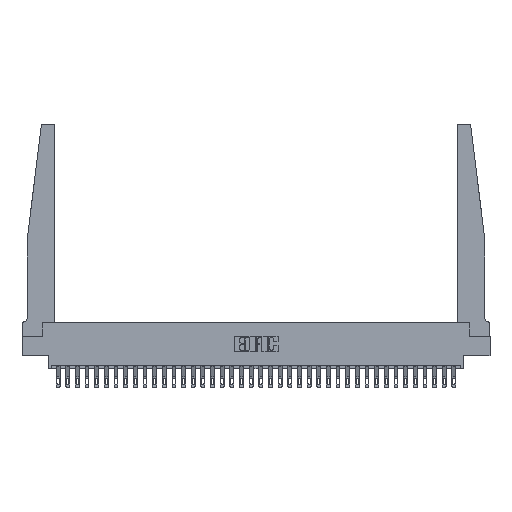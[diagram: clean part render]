
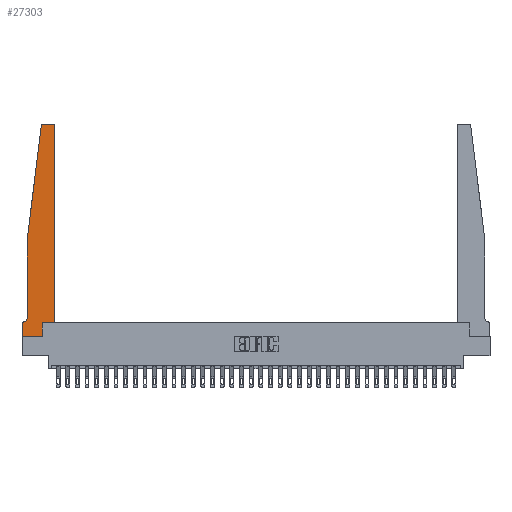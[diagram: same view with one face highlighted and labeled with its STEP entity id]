
A CAD part, top view. The second image highlights one B-rep face of the part: STEP entity #27303.
In plain terms, the highlighted planar face has unit normal (0, 0, 1).
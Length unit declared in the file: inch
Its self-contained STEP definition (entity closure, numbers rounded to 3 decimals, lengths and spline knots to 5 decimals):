
#251 = DIRECTION ( 'NONE',  ( -1., 0., 0. ) ) ;
#443 = ORIENTED_EDGE ( 'NONE', *, *, #30483, .T. ) ;
#712 = VECTOR ( 'NONE', #25133, 39.37008 ) ;
#1292 = ORIENTED_EDGE ( 'NONE', *, *, #17902, .T. ) ;
#2018 = CARTESIAN_POINT ( 'NONE',  ( 0.27653, 2.72, 0.37 ) ) ;
#2339 = DIRECTION ( 'NONE',  ( 0., 0., 1. ) ) ;
#2345 = LINE ( 'NONE', #12556, #712 ) ;
#2623 = LINE ( 'NONE', #23044, #21802 ) ;
#2804 = CARTESIAN_POINT ( 'NONE',  ( 0.27653, 2.75, 0.37 ) ) ;
#2879 = EDGE_CURVE ( 'NONE', #19835, #14535, #21771, .T. ) ;
#3100 = EDGE_CURVE ( 'NONE', #9063, #32251, #10012, .T. ) ;
#3103 = VECTOR ( 'NONE', #7460, 39.37008 ) ;
#3118 = CARTESIAN_POINT ( 'NONE',  ( 0.425, 0.18, 0.37 ) ) ;
#3523 = VERTEX_POINT ( 'NONE', #20181 ) ;
#3571 = FACE_OUTER_BOUND ( 'NONE', #21471, .T. ) ;
#3615 = LINE ( 'NONE', #13838, #16624 ) ;
#3735 = VECTOR ( 'NONE', #15206, 39.37008 ) ;
#4100 = DIRECTION ( 'NONE',  ( 1., 0., 0. ) ) ;
#4195 = ORIENTED_EDGE ( 'NONE', *, *, #2879, .T. ) ;
#4734 = EDGE_CURVE ( 'NONE', #32251, #16975, #20348, .T. ) ;
#4829 = EDGE_CURVE ( 'NONE', #31759, #8636, #2623, .T. ) ;
#5048 = CARTESIAN_POINT ( 'NONE',  ( 0.24675, 2.72367, 0.37 ) ) ;
#5418 = ORIENTED_EDGE ( 'NONE', *, *, #32273, .T. ) ;
#5441 = ORIENTED_EDGE ( 'NONE', *, *, #25520, .T. ) ;
#6023 = CARTESIAN_POINT ( 'NONE',  ( 0.2605, 0., 0.37 ) ) ;
#6103 = CARTESIAN_POINT ( 'NONE',  ( 0., 0., 0.37 ) ) ;
#6247 = DIRECTION ( 'NONE',  ( 1., 0., 0. ) ) ;
#6386 = CIRCLE ( 'NONE', #14946, 0.05 ) ;
#7021 = ORIENTED_EDGE ( 'NONE', *, *, #22419, .T. ) ;
#7460 = DIRECTION ( 'NONE',  ( 0., -1., 0. ) ) ;
#8636 = VERTEX_POINT ( 'NONE', #30446 ) ;
#8639 = DIRECTION ( 'NONE',  ( 0., 1., 0. ) ) ;
#8649 = CIRCLE ( 'NONE', #16198, 0.03 ) ;
#8762 = CARTESIAN_POINT ( 'NONE',  ( 0., 0.1875, 0.37 ) ) ;
#9031 = VECTOR ( 'NONE', #4100, 39.37008 ) ;
#9063 = VERTEX_POINT ( 'NONE', #5048 ) ;
#9319 = DIRECTION ( 'NONE',  ( -1., 0., 0. ) ) ;
#9564 = EDGE_CURVE ( 'NONE', #14535, #9063, #8649, .T. ) ;
#10012 = LINE ( 'NONE', #30470, #3735 ) ;
#10128 = DIRECTION ( 'NONE',  ( 0., 0., -1. ) ) ;
#10721 = VERTEX_POINT ( 'NONE', #28038 ) ;
#10940 = CARTESIAN_POINT ( 'NONE',  ( 0.395, 2.72, 0.37 ) ) ;
#12046 = CARTESIAN_POINT ( 'NONE',  ( 0.25, 2.75, 0.37 ) ) ;
#12157 = CARTESIAN_POINT ( 'NONE',  ( 0.065, 0.1875, 0.37 ) ) ;
#12234 = DIRECTION ( 'NONE',  ( 1., 0., 0. ) ) ;
#12323 = CARTESIAN_POINT ( 'NONE',  ( 0., 0., 0.37 ) ) ;
#12491 = CARTESIAN_POINT ( 'NONE',  ( 0.015, 0.2375, 0.37 ) ) ;
#12556 = CARTESIAN_POINT ( 'NONE',  ( 0.425, 0.18, 0.37 ) ) ;
#12563 = CARTESIAN_POINT ( 'NONE',  ( 0.395, 2.75, 0.37 ) ) ;
#13838 = CARTESIAN_POINT ( 'NONE',  ( 0., 0., 0.37 ) ) ;
#13849 = ORIENTED_EDGE ( 'NONE', *, *, #4829, .T. ) ;
#14535 = VERTEX_POINT ( 'NONE', #2804 ) ;
#14572 = DIRECTION ( 'NONE',  ( -1., 0., 0. ) ) ;
#14625 = ORIENTED_EDGE ( 'NONE', *, *, #17538, .T. ) ;
#14946 = AXIS2_PLACEMENT_3D ( 'NONE', #12491, #10128, #251 ) ;
#15206 = DIRECTION ( 'NONE',  ( -0.122, -0.992, 0. ) ) ;
#15298 = DIRECTION ( 'NONE',  ( 0., 0., 1. ) ) ;
#15834 = LINE ( 'NONE', #3118, #21204 ) ;
#16198 = AXIS2_PLACEMENT_3D ( 'NONE', #2018, #2339, #12234 ) ;
#16624 = VECTOR ( 'NONE', #19010, 39.37008 ) ;
#16975 = VERTEX_POINT ( 'NONE', #20726 ) ;
#17502 = CIRCLE ( 'NONE', #26073, 0.03 ) ;
#17538 = EDGE_CURVE ( 'NONE', #28084, #3523, #15834, .T. ) ;
#17902 = EDGE_CURVE ( 'NONE', #3523, #19835, #17502, .T. ) ;
#18138 = DIRECTION ( 'NONE',  ( 1., 0., 0. ) ) ;
#18936 = VERTEX_POINT ( 'NONE', #12323 ) ;
#19010 = DIRECTION ( 'NONE',  ( 0., -1., 0. ) ) ;
#19142 = PLANE ( 'NONE',  #25193 ) ;
#19619 = VECTOR ( 'NONE', #14572, 39.37008 ) ;
#19635 = CARTESIAN_POINT ( 'NONE',  ( 0.015, 0.1875, 0.37 ) ) ;
#19835 = VERTEX_POINT ( 'NONE', #12563 ) ;
#20181 = CARTESIAN_POINT ( 'NONE',  ( 0.425, 2.72, 0.37 ) ) ;
#20348 = LINE ( 'NONE', #20517, #3103 ) ;
#20517 = CARTESIAN_POINT ( 'NONE',  ( 0.065, 1.25, 0.37 ) ) ;
#20726 = CARTESIAN_POINT ( 'NONE',  ( 0.065, 0.2375, 0.37 ) ) ;
#20914 = LINE ( 'NONE', #6103, #9031 ) ;
#21204 = VECTOR ( 'NONE', #23559, 39.37008 ) ;
#21471 = EDGE_LOOP ( 'NONE', ( #4195, #22852, #27718, #32979, #5441, #5418, #24728, #7021, #13849, #443, #14625, #1292 ) ) ;
#21771 = LINE ( 'NONE', #12046, #19619 ) ;
#21802 = VECTOR ( 'NONE', #8639, 39.37008 ) ;
#22419 = EDGE_CURVE ( 'NONE', #18936, #31759, #20914, .T. ) ;
#22852 = ORIENTED_EDGE ( 'NONE', *, *, #9564, .T. ) ;
#23044 = CARTESIAN_POINT ( 'NONE',  ( 0.2605, 0.18, 0.37 ) ) ;
#23559 = DIRECTION ( 'NONE',  ( 0., 1., 0. ) ) ;
#24728 = ORIENTED_EDGE ( 'NONE', *, *, #26796, .T. ) ;
#25060 = CARTESIAN_POINT ( 'NONE',  ( 0.065, 1.25, 0.37 ) ) ;
#25133 = DIRECTION ( 'NONE',  ( 1., 0., 0. ) ) ;
#25193 = AXIS2_PLACEMENT_3D ( 'NONE', #8762, #29209, #6247 ) ;
#25520 = EDGE_CURVE ( 'NONE', #16975, #28592, #6386, .T. ) ;
#26073 = AXIS2_PLACEMENT_3D ( 'NONE', #10940, #15298, #18138 ) ;
#26616 = CARTESIAN_POINT ( 'NONE',  ( 0.425, 0.18, 0.37 ) ) ;
#26796 = EDGE_CURVE ( 'NONE', #10721, #18936, #3615, .T. ) ;
#27303 = ADVANCED_FACE ( 'NONE', ( #3571 ), #19142, .T. ) ;
#27718 = ORIENTED_EDGE ( 'NONE', *, *, #3100, .T. ) ;
#28038 = CARTESIAN_POINT ( 'NONE',  ( 0., 0.1875, 0.37 ) ) ;
#28084 = VERTEX_POINT ( 'NONE', #26616 ) ;
#28592 = VERTEX_POINT ( 'NONE', #19635 ) ;
#29209 = DIRECTION ( 'NONE',  ( 0., 0., 1. ) ) ;
#29952 = LINE ( 'NONE', #12157, #32807 ) ;
#30446 = CARTESIAN_POINT ( 'NONE',  ( 0.2605, 0.18, 0.37 ) ) ;
#30470 = CARTESIAN_POINT ( 'NONE',  ( 0.065, 1.25, 0.37 ) ) ;
#30483 = EDGE_CURVE ( 'NONE', #8636, #28084, #2345, .T. ) ;
#31759 = VERTEX_POINT ( 'NONE', #6023 ) ;
#32251 = VERTEX_POINT ( 'NONE', #25060 ) ;
#32273 = EDGE_CURVE ( 'NONE', #28592, #10721, #29952, .T. ) ;
#32807 = VECTOR ( 'NONE', #9319, 39.37008 ) ;
#32979 = ORIENTED_EDGE ( 'NONE', *, *, #4734, .T. ) ;
